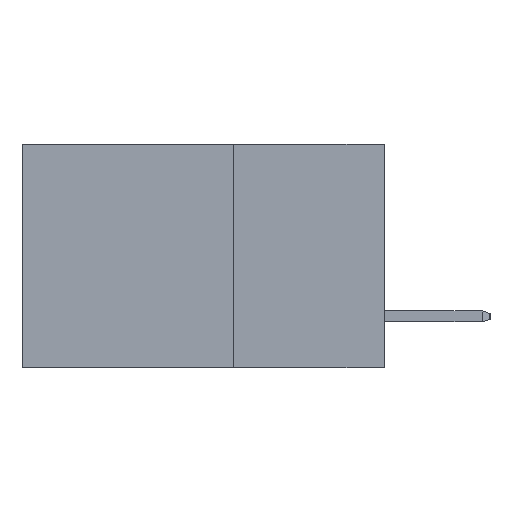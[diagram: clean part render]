
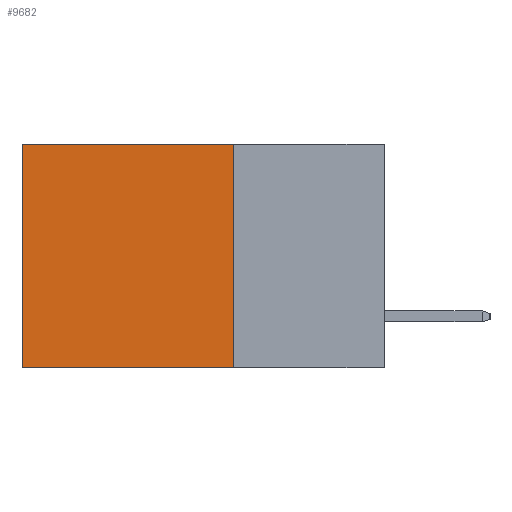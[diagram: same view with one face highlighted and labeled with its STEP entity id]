
A CAD part, left-side view. The second image highlights one B-rep face of the part: STEP entity #9682.
In plain terms, the highlighted planar face has unit normal (-1, 0, 0).
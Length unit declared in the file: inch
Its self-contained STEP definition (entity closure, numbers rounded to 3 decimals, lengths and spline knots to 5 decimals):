
#173 = CARTESIAN_POINT ( 'NONE',  ( 0.2615, 0.25, -0.37 ) ) ;
#1021 = LINE ( 'NONE', #15797, #4740 ) ;
#1171 = ORIENTED_EDGE ( 'NONE', *, *, #15062, .T. ) ;
#1385 = CARTESIAN_POINT ( 'NONE',  ( 0.2615, 0.25, 0. ) ) ;
#1573 = EDGE_CURVE ( 'NONE', #7726, #10386, #1021, .T. ) ;
#1597 = EDGE_CURVE ( 'NONE', #14322, #10386, #15245, .T. ) ;
#2069 = ORIENTED_EDGE ( 'NONE', *, *, #1597, .T. ) ;
#2224 = ORIENTED_EDGE ( 'NONE', *, *, #10094, .F. ) ;
#2525 = CARTESIAN_POINT ( 'NONE',  ( 0.2615, 0.25, -0.37 ) ) ;
#3543 = CARTESIAN_POINT ( 'NONE',  ( 0.2615, 0.25, -0.37 ) ) ;
#4078 = FACE_OUTER_BOUND ( 'NONE', #13226, .T. ) ;
#4476 = LINE ( 'NONE', #1385, #11438 ) ;
#4505 = LINE ( 'NONE', #3543, #14597 ) ;
#4740 = VECTOR ( 'NONE', #7706, 39.37008 ) ;
#4864 = CARTESIAN_POINT ( 'NONE',  ( 0.2615, 0.6, -0.37 ) ) ;
#4937 = DIRECTION ( 'NONE',  ( 0., 0., -1. ) ) ;
#6140 = AXIS2_PLACEMENT_3D ( 'NONE', #2525, #16223, #8135 ) ;
#6216 = DIRECTION ( 'NONE',  ( 0., 0., -1. ) ) ;
#6723 = PLANE ( 'NONE',  #6140 ) ;
#6826 = CARTESIAN_POINT ( 'NONE',  ( 0.2615, 0.6, -0.37 ) ) ;
#7706 = DIRECTION ( 'NONE',  ( 0., 1., 0. ) ) ;
#7726 = VERTEX_POINT ( 'NONE', #173 ) ;
#8135 = DIRECTION ( 'NONE',  ( 0., 0., -1. ) ) ;
#8451 = VECTOR ( 'NONE', #6216, 39.37008 ) ;
#9682 = ADVANCED_FACE ( 'NONE', ( #4078 ), #6723, .F. ) ;
#10094 = EDGE_CURVE ( 'NONE', #10936, #7726, #4505, .T. ) ;
#10386 = VERTEX_POINT ( 'NONE', #6826 ) ;
#10736 = CARTESIAN_POINT ( 'NONE',  ( 0.2615, 0.25, 0. ) ) ;
#10936 = VERTEX_POINT ( 'NONE', #10736 ) ;
#11438 = VECTOR ( 'NONE', #13809, 39.37008 ) ;
#13226 = EDGE_LOOP ( 'NONE', ( #2069, #17737, #2224, #1171 ) ) ;
#13809 = DIRECTION ( 'NONE',  ( 0., 1., 0. ) ) ;
#14322 = VERTEX_POINT ( 'NONE', #16535 ) ;
#14597 = VECTOR ( 'NONE', #4937, 39.37008 ) ;
#15062 = EDGE_CURVE ( 'NONE', #10936, #14322, #4476, .T. ) ;
#15245 = LINE ( 'NONE', #4864, #8451 ) ;
#15797 = CARTESIAN_POINT ( 'NONE',  ( 0.2615, 0.25, -0.37 ) ) ;
#16223 = DIRECTION ( 'NONE',  ( 1., 0., 0. ) ) ;
#16535 = CARTESIAN_POINT ( 'NONE',  ( 0.2615, 0.6, 0. ) ) ;
#17737 = ORIENTED_EDGE ( 'NONE', *, *, #1573, .F. ) ;
